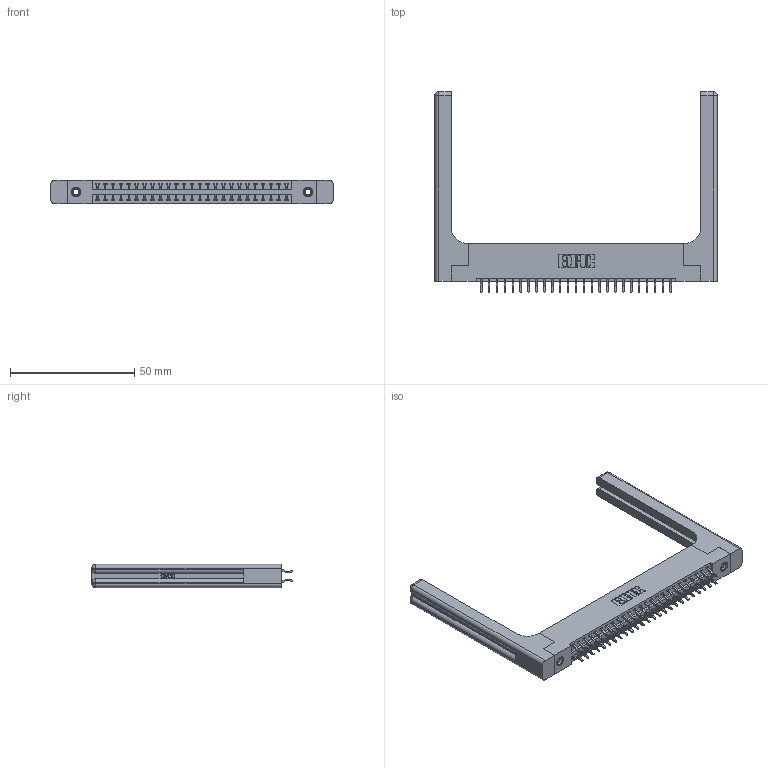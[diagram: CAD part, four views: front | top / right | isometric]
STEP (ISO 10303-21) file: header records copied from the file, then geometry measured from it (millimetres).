
FILE_DESCRIPTION (( 'STEP AP203' ), '1' );
FILE_NAME ('396-050-556-258.STEP', '2019-10-30T13:18:13', ( '' ), ( '' ), 'SwSTEP 2.0', 'SolidWorks 2016', '' );
FILE_SCHEMA (( 'CONFIG_CONTROL_DESIGN' ));
Length unit declared in the file: inch
Products named in the file (5): 346-220-058_345-220-058; 345-292-001_556 Tail; 345-250-001_345-250-001-102; 346 Part_Flush Mounting Lugs - 0.156 Dia-TH; 396-050-556-258
Assembly tree (55 placements, depth 2):
  396-050-556-258
    346 Part_Flush Mounting Lugs - 0.156 Dia-TH
    345-292-001_556 Tail  x50
    345-250-001_345-250-001-102  x2
    346-220-058_345-220-058  x2
Bounding box: 113.44 x 80.53 x 9.4 mm (x, y, z)
Volume: 18421.7 mm3; surface area: 19679.6 mm2
Topology: 55 solids, 55 shells, 3278 faces, 9645 edges, 6342 vertices
Faces by surface type: plane 2174, cylinder 1044, bspline 36, cone 12, sphere 8, torus 4
Entity records: 24006 total; most frequent: CARTESIAN_POINT 5001, ORIENTED_EDGE 3720, DIRECTION 3380, EDGE_CURVE 1860, LINE 1528, VECTOR 1528, VERTEX_POINT 1230, AXIS2_PLACEMENT_3D 926
